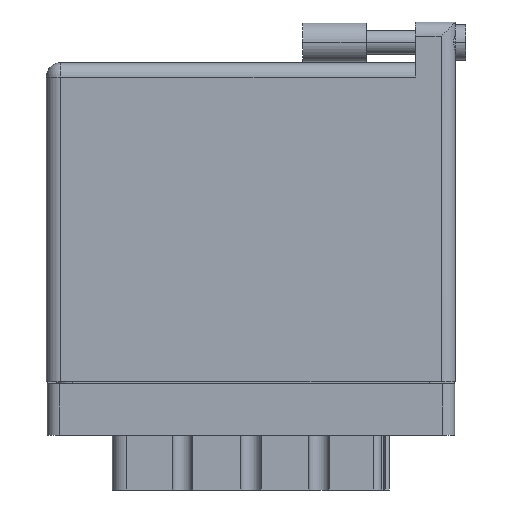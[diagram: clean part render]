
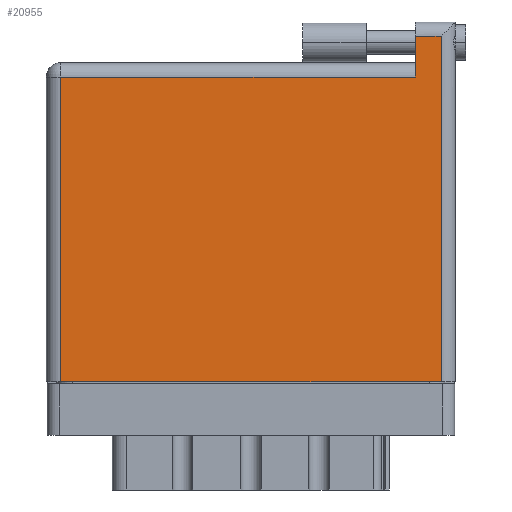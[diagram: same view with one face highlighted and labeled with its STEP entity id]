
A CAD part, front view. The second image highlights one B-rep face of the part: STEP entity #20955.
In plain terms, the highlighted face is planar.
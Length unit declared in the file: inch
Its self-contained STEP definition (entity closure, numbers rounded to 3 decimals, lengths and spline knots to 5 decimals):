
#311 = ORIENTED_EDGE ( 'NONE', *, *, #3950, .T. ) ;
#2571 = ORIENTED_EDGE ( 'NONE', *, *, #39965, .T. ) ;
#3769 = LINE ( 'NONE', #16768, #6749 ) ;
#3950 = EDGE_CURVE ( 'NONE', #5508, #8105, #40330, .T. ) ;
#4444 = VERTEX_POINT ( 'NONE', #13358 ) ;
#4877 = CARTESIAN_POINT ( 'NONE',  ( 0.07, 0., 0. ) ) ;
#5015 = DIRECTION ( 'NONE',  ( 0., -1., 0. ) ) ;
#5116 = CARTESIAN_POINT ( 'NONE',  ( 0., 1.566, 0. ) ) ;
#5508 = VERTEX_POINT ( 'NONE', #21994 ) ;
#5910 = VECTOR ( 'NONE', #37920, 39.37008 ) ;
#6749 = VECTOR ( 'NONE', #36136, 39.37008 ) ;
#7208 = VECTOR ( 'NONE', #15643, 39.37008 ) ;
#7882 = DIRECTION ( 'NONE',  ( -1., 0., 0. ) ) ;
#8105 = VERTEX_POINT ( 'NONE', #29148 ) ;
#11197 = ORIENTED_EDGE ( 'NONE', *, *, #11663, .T. ) ;
#11663 = EDGE_CURVE ( 'NONE', #19194, #15386, #3769, .T. ) ;
#13358 = CARTESIAN_POINT ( 'NONE',  ( 0.07, 0., 0. ) ) ;
#15386 = VERTEX_POINT ( 'NONE', #37009 ) ;
#15641 = VECTOR ( 'NONE', #38206, 39.37008 ) ;
#15643 = DIRECTION ( 'NONE',  ( -1., 0., 0. ) ) ;
#16676 = CARTESIAN_POINT ( 'NONE',  ( 1.811, 1.696, 0. ) ) ;
#16768 = CARTESIAN_POINT ( 'NONE',  ( 1.938, 1.766, 0. ) ) ;
#17593 = DIRECTION ( 'NONE',  ( 0., 0., -1. ) ) ;
#17842 = EDGE_CURVE ( 'NONE', #8105, #4444, #40006, .T. ) ;
#19194 = VERTEX_POINT ( 'NONE', #28920 ) ;
#19358 = VERTEX_POINT ( 'NONE', #16676 ) ;
#19508 = FACE_OUTER_BOUND ( 'NONE', #35624, .T. ) ;
#19986 = DIRECTION ( 'NONE',  ( 0., -1., 0. ) ) ;
#20955 = ADVANCED_FACE ( 'NONE', ( #19508 ), #39246, .F. ) ;
#21861 = ORIENTED_EDGE ( 'NONE', *, *, #17842, .T. ) ;
#21994 = CARTESIAN_POINT ( 'NONE',  ( 1.811, 1.496, 0. ) ) ;
#22074 = CARTESIAN_POINT ( 'NONE',  ( 0., 1.696, 0. ) ) ;
#25638 = CARTESIAN_POINT ( 'NONE',  ( 0., 1.496, 0. ) ) ;
#28608 = VECTOR ( 'NONE', #5015, 39.37008 ) ;
#28672 = EDGE_CURVE ( 'NONE', #15386, #19358, #39359, .T. ) ;
#28920 = CARTESIAN_POINT ( 'NONE',  ( 1.938, 0., 0. ) ) ;
#29111 = ORIENTED_EDGE ( 'NONE', *, *, #32556, .T. ) ;
#29134 = LINE ( 'NONE', #31664, #5910 ) ;
#29148 = CARTESIAN_POINT ( 'NONE',  ( 0.07, 1.496, 0. ) ) ;
#30969 = VECTOR ( 'NONE', #19986, 39.37008 ) ;
#31664 = CARTESIAN_POINT ( 'NONE',  ( 0., 0., 0. ) ) ;
#32556 = EDGE_CURVE ( 'NONE', #4444, #19194, #29134, .T. ) ;
#34424 = LINE ( 'NONE', #35992, #30969 ) ;
#35624 = EDGE_LOOP ( 'NONE', ( #29111, #11197, #39060, #2571, #311, #21861 ) ) ;
#35992 = CARTESIAN_POINT ( 'NONE',  ( 1.811, 1.766, 0. ) ) ;
#36136 = DIRECTION ( 'NONE',  ( 0., 1., 0. ) ) ;
#37009 = CARTESIAN_POINT ( 'NONE',  ( 1.938, 1.696, 0. ) ) ;
#37920 = DIRECTION ( 'NONE',  ( 1., 0., 0. ) ) ;
#38206 = DIRECTION ( 'NONE',  ( -1., 0., 0. ) ) ;
#39060 = ORIENTED_EDGE ( 'NONE', *, *, #28672, .T. ) ;
#39246 = PLANE ( 'NONE',  #40329 ) ;
#39359 = LINE ( 'NONE', #22074, #7208 ) ;
#39965 = EDGE_CURVE ( 'NONE', #19358, #5508, #34424, .T. ) ;
#40006 = LINE ( 'NONE', #4877, #28608 ) ;
#40329 = AXIS2_PLACEMENT_3D ( 'NONE', #5116, #17593, #7882 ) ;
#40330 = LINE ( 'NONE', #25638, #15641 ) ;
